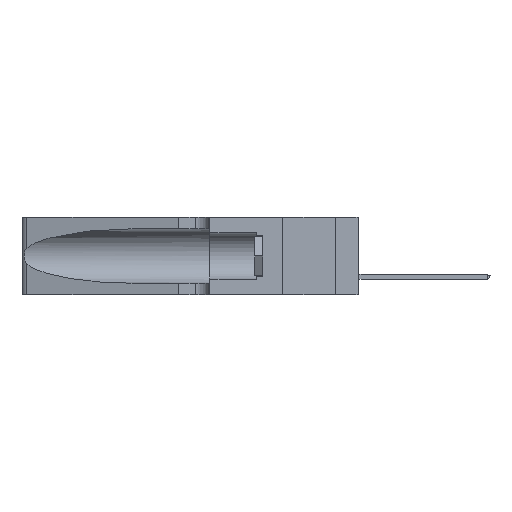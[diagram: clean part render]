
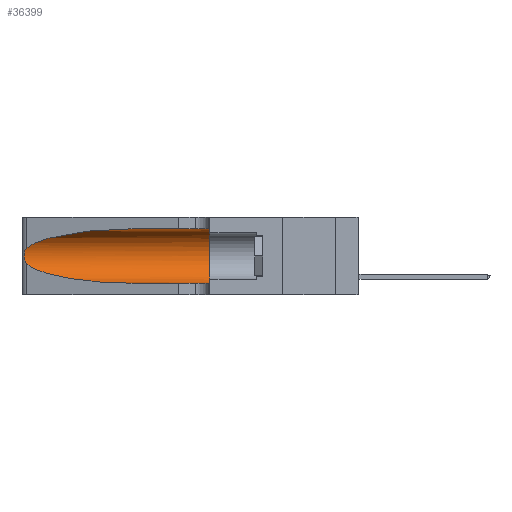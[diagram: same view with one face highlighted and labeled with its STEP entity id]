
A CAD part, left-side view. The second image highlights one B-rep face of the part: STEP entity #36399.
In plain terms, the highlighted cylindrical face has radius 3.308 mm (diameter 6.617 mm), a partial arc.
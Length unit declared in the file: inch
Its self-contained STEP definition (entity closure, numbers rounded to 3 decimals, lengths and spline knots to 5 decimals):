
#164 = EDGE_CURVE ( 'NONE', #11855, #28032, #44811, .T. ) ;
#305 = CARTESIAN_POINT ( 'NONE',  ( 0.18966, 0.96281, 0.31525 ) ) ;
#358 = CARTESIAN_POINT ( 'NONE',  ( 0.26017, 1.23833, 0.17102 ) ) ;
#772 = CARTESIAN_POINT ( 'NONE',  ( 0.25487, 1.22718, 0.14631 ) ) ;
#1151 = CARTESIAN_POINT ( 'NONE',  ( 0.25487, 1.22718, 0.22369 ) ) ;
#1549 = CARTESIAN_POINT ( 'NONE',  ( 0.1305, 1.61858, 0.185 ) ) ;
#1677 = EDGE_CURVE ( 'NONE', #28032, #13629, #30996, .T. ) ;
#3254 = CARTESIAN_POINT ( 'NONE',  ( 0.25787, 1.23484, 0.2124 ) ) ;
#4303 = CARTESIAN_POINT ( 'NONE',  ( 0.2373, 1.15595, 0.28018 ) ) ;
#4322 = CYLINDRICAL_SURFACE ( 'NONE', #8948, 0.13025 ) ;
#4612 = VERTEX_POINT ( 'NONE', #16964 ) ;
#5688 = LINE ( 'NONE', #12227, #7976 ) ;
#6036 = ORIENTED_EDGE ( 'NONE', *, *, #1677, .F. ) ;
#7052 = CARTESIAN_POINT ( 'NONE',  ( 0.25639, 1.23186, 0.15144 ) ) ;
#7224 = CARTESIAN_POINT ( 'NONE',  ( 0.25555, 1.22993, 0.14849 ) ) ;
#7578 = CARTESIAN_POINT ( 'NONE',  ( 0.18966, 0.96281, 0.05475 ) ) ;
#7976 = VECTOR ( 'NONE', #16329, 39.37008 ) ;
#8746 = DIRECTION ( 'NONE',  ( 0., -1., 0. ) ) ;
#8894 = FACE_OUTER_BOUND ( 'NONE', #31113, .T. ) ;
#8948 = AXIS2_PLACEMENT_3D ( 'NONE', #1549, #8746, #30815 ) ;
#10045 = DIRECTION ( 'NONE',  ( 0., 0., 1. ) ) ;
#10197 = DIRECTION ( 'NONE',  ( 0., 1., 0. ) ) ;
#11327 = EDGE_CURVE ( 'NONE', #40434, #15898, #42446, .T. ) ;
#11855 = VERTEX_POINT ( 'NONE', #18096 ) ;
#12227 = CARTESIAN_POINT ( 'NONE',  ( 0.1305, 1.61858, 0.05475 ) ) ;
#13286 =( BOUNDED_CURVE ( )  B_SPLINE_CURVE ( 3, ( #18620, #29778, #7578, #37416 ),
 .UNSPECIFIED., .F., .F. ) 
 B_SPLINE_CURVE_WITH_KNOTS ( ( 4, 4 ),
 ( 3.44316, 4.71239 ),
 .UNSPECIFIED. ) 
 CURVE ( )  GEOMETRIC_REPRESENTATION_ITEM ( )  RATIONAL_B_SPLINE_CURVE ( ( 1., 0.87, 0.87, 1. ) ) 
 REPRESENTATION_ITEM ( '' )  );
#13572 = CARTESIAN_POINT ( 'NONE',  ( 0.1305, 0.35, 0.185 ) ) ;
#13629 = VERTEX_POINT ( 'NONE', #16682 ) ;
#14278 = CARTESIAN_POINT ( 'NONE',  ( 0.26075, 1.23896, 0.178 ) ) ;
#14844 = CARTESIAN_POINT ( 'NONE',  ( 0.1305, 0.35, 0.31525 ) ) ;
#15898 = VERTEX_POINT ( 'NONE', #772 ) ;
#16329 = DIRECTION ( 'NONE',  ( 0., -1., 0. ) ) ;
#16682 = CARTESIAN_POINT ( 'NONE',  ( 0.1305, 0.35, 0.05475 ) ) ;
#16964 = CARTESIAN_POINT ( 'NONE',  ( 0.1305, 0.72297, 0.05475 ) ) ;
#18096 = CARTESIAN_POINT ( 'NONE',  ( 0.1305, 0.72297, 0.31525 ) ) ;
#18560 = CARTESIAN_POINT ( 'NONE',  ( 0.1305, 0.72297, 0.31525 ) ) ;
#18620 = CARTESIAN_POINT ( 'NONE',  ( 0.25487, 1.22718, 0.14631 ) ) ;
#21234 = CARTESIAN_POINT ( 'NONE',  ( 0.25854, 1.2359, 0.20912 ) ) ;
#21555 = CARTESIAN_POINT ( 'NONE',  ( 0.25555, 1.22994, 0.2215 ) ) ;
#22028 = CARTESIAN_POINT ( 'NONE',  ( 0.25487, 1.22718, 0.14631 ) ) ;
#23309 = CARTESIAN_POINT ( 'NONE',  ( 0.1305, 1.61858, 0.31525 ) ) ;
#24386 = EDGE_CURVE ( 'NONE', #4612, #13629, #5688, .T. ) ;
#24805 =( BOUNDED_CURVE ( )  B_SPLINE_CURVE ( 3, ( #18560, #305, #4303, #33398 ),
 .UNSPECIFIED., .F., .F. ) 
 B_SPLINE_CURVE_WITH_KNOTS ( ( 4, 4 ),
 ( 1.5708, 2.84003 ),
 .UNSPECIFIED. ) 
 CURVE ( )  GEOMETRIC_REPRESENTATION_ITEM ( )  RATIONAL_B_SPLINE_CURVE ( ( 1., 0.87, 0.87, 1. ) ) 
 REPRESENTATION_ITEM ( '' )  );
#25096 = CARTESIAN_POINT ( 'NONE',  ( 0.25639, 1.23184, 0.21858 ) ) ;
#27633 = ORIENTED_EDGE ( 'NONE', *, *, #38788, .T. ) ;
#28032 = VERTEX_POINT ( 'NONE', #14844 ) ;
#29034 = ORIENTED_EDGE ( 'NONE', *, *, #11327, .T. ) ;
#29101 = CARTESIAN_POINT ( 'NONE',  ( 0.25789, 1.23486, 0.15765 ) ) ;
#29356 = VECTOR ( 'NONE', #45119, 39.37008 ) ;
#29778 = CARTESIAN_POINT ( 'NONE',  ( 0.2373, 1.15595, 0.08982 ) ) ;
#30815 = DIRECTION ( 'NONE',  ( 0., 0., -1. ) ) ;
#30996 = CIRCLE ( 'NONE', #47093, 0.13025 ) ;
#31113 = EDGE_LOOP ( 'NONE', ( #27633, #29034, #39930, #44120, #6036, #33099 ) ) ;
#32037 = EDGE_CURVE ( 'NONE', #15898, #4612, #13286, .T. ) ;
#33099 = ORIENTED_EDGE ( 'NONE', *, *, #164, .F. ) ;
#33398 = CARTESIAN_POINT ( 'NONE',  ( 0.25487, 1.22718, 0.22369 ) ) ;
#36322 = CARTESIAN_POINT ( 'NONE',  ( 0.26075, 1.23896, 0.19203 ) ) ;
#36399 = ADVANCED_FACE ( 'NONE', ( #8894 ), #4322, .F. ) ;
#37118 = CARTESIAN_POINT ( 'NONE',  ( 0.25856, 1.23593, 0.16098 ) ) ;
#37416 = CARTESIAN_POINT ( 'NONE',  ( 0.1305, 0.72297, 0.05475 ) ) ;
#38788 = EDGE_CURVE ( 'NONE', #11855, #40434, #24805, .T. ) ;
#39528 = CARTESIAN_POINT ( 'NONE',  ( 0.25487, 1.22718, 0.22369 ) ) ;
#39930 = ORIENTED_EDGE ( 'NONE', *, *, #32037, .T. ) ;
#40434 = VERTEX_POINT ( 'NONE', #1151 ) ;
#42446 = B_SPLINE_CURVE_WITH_KNOTS ( 'NONE', 3,
 ( #39528, #21555, #25096, #3254, #21234, #46882, #36322, #14278, #358, #37118, #29101, #7052, #7224, #22028 ),
 .UNSPECIFIED., .F., .F.,
 ( 4, 2, 2, 2, 2, 2, 4 ),
 ( 0., 0.00027, 0.00053, 0.00107, 0.0016, 0.00187, 0.00214 ),
 .UNSPECIFIED. ) ;
#44120 = ORIENTED_EDGE ( 'NONE', *, *, #24386, .T. ) ;
#44811 = LINE ( 'NONE', #23309, #29356 ) ;
#45119 = DIRECTION ( 'NONE',  ( 0., -1., 0. ) ) ;
#46882 = CARTESIAN_POINT ( 'NONE',  ( 0.26018, 1.23835, 0.19895 ) ) ;
#47093 = AXIS2_PLACEMENT_3D ( 'NONE', #13572, #10197, #10045 ) ;
